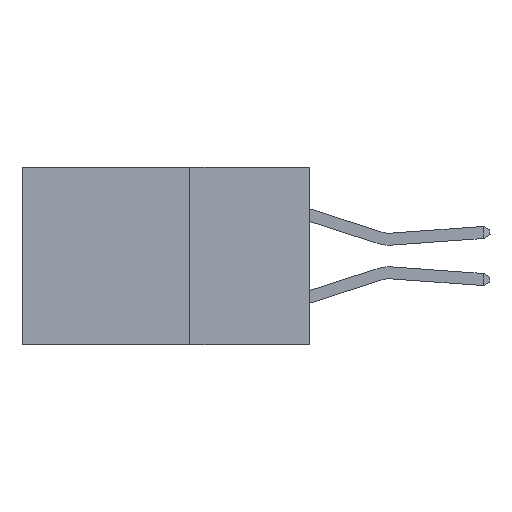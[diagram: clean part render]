
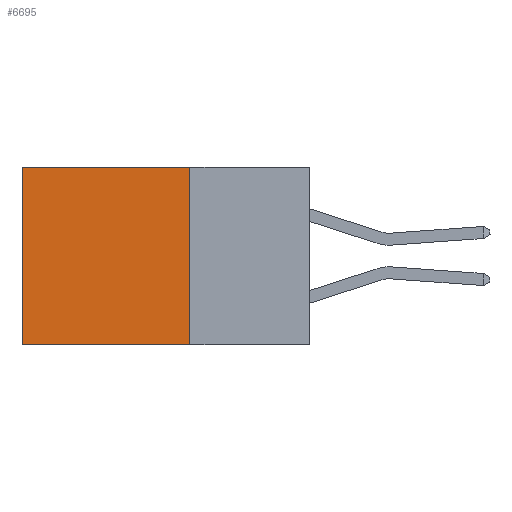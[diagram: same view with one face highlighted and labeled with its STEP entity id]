
A CAD part, left-side view. The second image highlights one B-rep face of the part: STEP entity #6695.
In plain terms, the highlighted planar face has unit normal (-1, 0, 0).
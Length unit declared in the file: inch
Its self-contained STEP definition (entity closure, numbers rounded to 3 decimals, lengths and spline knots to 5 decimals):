
#196 = PLANE ( 'NONE',  #7121 ) ;
#1450 = DIRECTION ( 'NONE',  ( 1., 0., 0. ) ) ;
#1597 = LINE ( 'NONE', #8670, #11370 ) ;
#3198 = VERTEX_POINT ( 'NONE', #14889 ) ;
#3545 = LINE ( 'NONE', #10008, #9898 ) ;
#4024 = CARTESIAN_POINT ( 'NONE',  ( 0.298, 0.25, -0.37 ) ) ;
#4228 = DIRECTION ( 'NONE',  ( 0., 0., -1. ) ) ;
#4800 = DIRECTION ( 'NONE',  ( 0., 1., 0. ) ) ;
#4839 = EDGE_LOOP ( 'NONE', ( #7052, #6369, #7584, #15970 ) ) ;
#5034 = CARTESIAN_POINT ( 'NONE',  ( 0.298, 0.25, 0. ) ) ;
#5180 = VECTOR ( 'NONE', #14301, 39.37008 ) ;
#5886 = VERTEX_POINT ( 'NONE', #8798 ) ;
#6369 = ORIENTED_EDGE ( 'NONE', *, *, #13786, .F. ) ;
#6593 = VERTEX_POINT ( 'NONE', #5034 ) ;
#6695 = ADVANCED_FACE ( 'NONE', ( #13249 ), #196, .F. ) ;
#7052 = ORIENTED_EDGE ( 'NONE', *, *, #9098, .T. ) ;
#7121 = AXIS2_PLACEMENT_3D ( 'NONE', #9037, #1450, #10346 ) ;
#7584 = ORIENTED_EDGE ( 'NONE', *, *, #10087, .F. ) ;
#8101 = CARTESIAN_POINT ( 'NONE',  ( 0.298, 0.25, -0.37 ) ) ;
#8670 = CARTESIAN_POINT ( 'NONE',  ( 0.298, 0.25, 0. ) ) ;
#8798 = CARTESIAN_POINT ( 'NONE',  ( 0.298, 0.6, -0.37 ) ) ;
#9037 = CARTESIAN_POINT ( 'NONE',  ( 0.298, 0.25, 0. ) ) ;
#9098 = EDGE_CURVE ( 'NONE', #3198, #5886, #13183, .T. ) ;
#9704 = VECTOR ( 'NONE', #4228, 39.37008 ) ;
#9898 = VECTOR ( 'NONE', #13886, 39.37008 ) ;
#10008 = CARTESIAN_POINT ( 'NONE',  ( 0.298, 0.25, 0. ) ) ;
#10087 = EDGE_CURVE ( 'NONE', #6593, #11128, #3545, .T. ) ;
#10346 = DIRECTION ( 'NONE',  ( 0., 0., -1. ) ) ;
#11128 = VERTEX_POINT ( 'NONE', #8101 ) ;
#11370 = VECTOR ( 'NONE', #4800, 39.37008 ) ;
#13183 = LINE ( 'NONE', #13245, #9704 ) ;
#13245 = CARTESIAN_POINT ( 'NONE',  ( 0.298, 0.6, 0. ) ) ;
#13249 = FACE_OUTER_BOUND ( 'NONE', #4839, .T. ) ;
#13786 = EDGE_CURVE ( 'NONE', #11128, #5886, #15840, .T. ) ;
#13886 = DIRECTION ( 'NONE',  ( 0., 0., -1. ) ) ;
#14301 = DIRECTION ( 'NONE',  ( 0., 1., 0. ) ) ;
#14889 = CARTESIAN_POINT ( 'NONE',  ( 0.298, 0.6, 0. ) ) ;
#15840 = LINE ( 'NONE', #4024, #5180 ) ;
#15970 = ORIENTED_EDGE ( 'NONE', *, *, #16452, .T. ) ;
#16452 = EDGE_CURVE ( 'NONE', #6593, #3198, #1597, .T. ) ;
